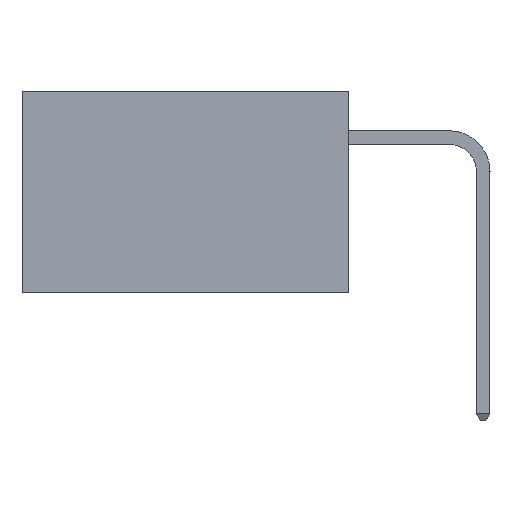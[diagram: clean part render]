
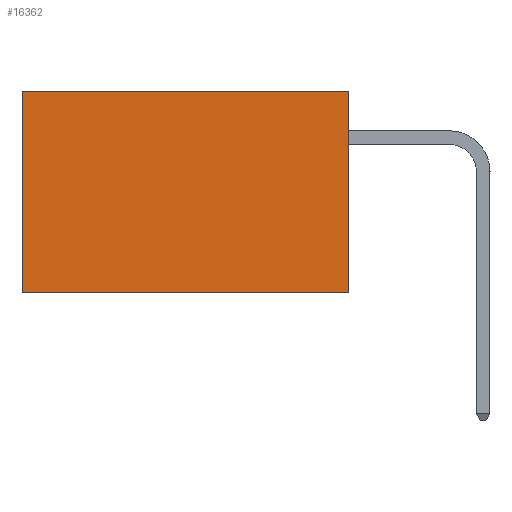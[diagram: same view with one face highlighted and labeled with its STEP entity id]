
A CAD part, left-side view. The second image highlights one B-rep face of the part: STEP entity #16362.
In plain terms, the highlighted planar face has unit normal (-1, 0, 0).
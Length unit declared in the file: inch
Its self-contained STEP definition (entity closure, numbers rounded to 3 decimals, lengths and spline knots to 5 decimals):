
#1630 = VERTEX_POINT ( 'NONE', #11545 ) ;
#2752 = CARTESIAN_POINT ( 'NONE',  ( 0.2875, 0., 0. ) ) ;
#3042 = EDGE_CURVE ( 'NONE', #1630, #5945, #6908, .T. ) ;
#3622 = EDGE_CURVE ( 'NONE', #15236, #4106, #15100, .T. ) ;
#3793 = ORIENTED_EDGE ( 'NONE', *, *, #8466, .T. ) ;
#4106 = VERTEX_POINT ( 'NONE', #25127 ) ;
#4657 = CARTESIAN_POINT ( 'NONE',  ( 0.2875, 0.6, -0.37 ) ) ;
#4864 = DIRECTION ( 'NONE',  ( 0., 0., -1. ) ) ;
#5945 = VERTEX_POINT ( 'NONE', #4657 ) ;
#5960 = VECTOR ( 'NONE', #18240, 39.37008 ) ;
#6908 = LINE ( 'NONE', #16168, #16888 ) ;
#7388 = CARTESIAN_POINT ( 'NONE',  ( 0.2875, 0., 0. ) ) ;
#7508 = DIRECTION ( 'NONE',  ( 0., 1., 0. ) ) ;
#7513 = EDGE_CURVE ( 'NONE', #15236, #1630, #13368, .T. ) ;
#7995 = VECTOR ( 'NONE', #17358, 39.37008 ) ;
#8466 = EDGE_CURVE ( 'NONE', #4106, #5945, #16631, .T. ) ;
#8972 = ORIENTED_EDGE ( 'NONE', *, *, #7513, .F. ) ;
#9523 = ORIENTED_EDGE ( 'NONE', *, *, #3622, .T. ) ;
#9880 = FACE_OUTER_BOUND ( 'NONE', #18573, .T. ) ;
#9952 = AXIS2_PLACEMENT_3D ( 'NONE', #2752, #16892, #4864 ) ;
#10396 = CARTESIAN_POINT ( 'NONE',  ( 0.2875, 0.6, 0. ) ) ;
#10999 = PLANE ( 'NONE',  #9952 ) ;
#11545 = CARTESIAN_POINT ( 'NONE',  ( 0.2875, 0., -0.37 ) ) ;
#13368 = LINE ( 'NONE', #25026, #7995 ) ;
#14369 = DIRECTION ( 'NONE',  ( 0., 1., 0. ) ) ;
#14465 = VECTOR ( 'NONE', #7508, 39.37008 ) ;
#15100 = LINE ( 'NONE', #7388, #14465 ) ;
#15236 = VERTEX_POINT ( 'NONE', #20629 ) ;
#16168 = CARTESIAN_POINT ( 'NONE',  ( 0.2875, 0., -0.37 ) ) ;
#16362 = ADVANCED_FACE ( 'NONE', ( #9880 ), #10999, .F. ) ;
#16631 = LINE ( 'NONE', #10396, #5960 ) ;
#16888 = VECTOR ( 'NONE', #14369, 39.37008 ) ;
#16892 = DIRECTION ( 'NONE',  ( 1., 0., 0. ) ) ;
#17358 = DIRECTION ( 'NONE',  ( 0., 0., -1. ) ) ;
#18240 = DIRECTION ( 'NONE',  ( 0., 0., -1. ) ) ;
#18573 = EDGE_LOOP ( 'NONE', ( #3793, #24167, #8972, #9523 ) ) ;
#20629 = CARTESIAN_POINT ( 'NONE',  ( 0.2875, 0., 0. ) ) ;
#24167 = ORIENTED_EDGE ( 'NONE', *, *, #3042, .F. ) ;
#25026 = CARTESIAN_POINT ( 'NONE',  ( 0.2875, 0., 0. ) ) ;
#25127 = CARTESIAN_POINT ( 'NONE',  ( 0.2875, 0.6, 0. ) ) ;
